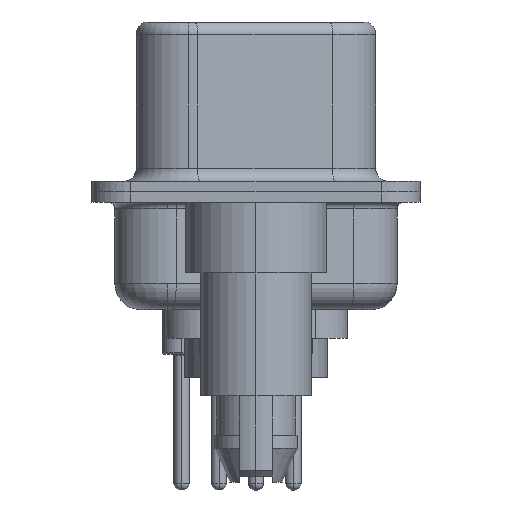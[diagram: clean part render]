
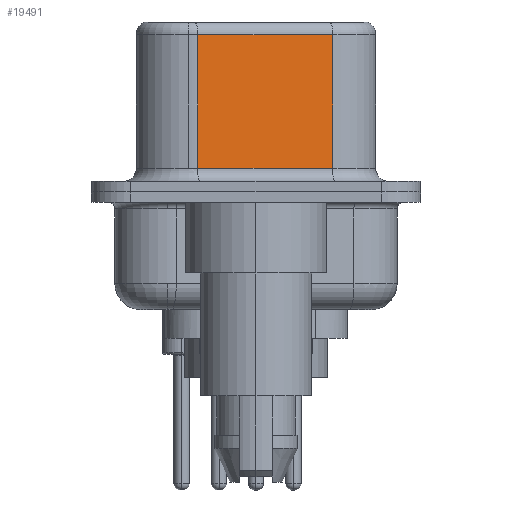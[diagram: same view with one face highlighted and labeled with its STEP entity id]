
A CAD part, left-side view. The second image highlights one B-rep face of the part: STEP entity #19491.
In plain terms, the highlighted planar face has unit normal (-0.985, -0.174, 0).
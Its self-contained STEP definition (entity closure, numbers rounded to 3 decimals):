
#1290 = VECTOR ( 'NONE', #22956, 1000. ) ;
#2112 = ORIENTED_EDGE ( 'NONE', *, *, #23496, .F. ) ;
#3891 = DIRECTION ( 'NONE',  ( 0., 0., -1. ) ) ;
#4011 = CARTESIAN_POINT ( 'NONE',  ( 4.585, -2.927, 6.02 ) ) ;
#4092 = VERTEX_POINT ( 'NONE', #12228 ) ;
#4845 = LINE ( 'NONE', #9576, #11020 ) ;
#5022 = EDGE_CURVE ( 'NONE', #10701, #4092, #4845, .T. ) ;
#5471 = LINE ( 'NONE', #13940, #19405 ) ;
#8380 = VERTEX_POINT ( 'NONE', #22483 ) ;
#9074 = CARTESIAN_POINT ( 'NONE',  ( 4.585, -2.927, 6.52 ) ) ;
#9576 = CARTESIAN_POINT ( 'NONE',  ( 4.585, -2.927, 6.02 ) ) ;
#10166 = EDGE_LOOP ( 'NONE', ( #2112, #16734, #15399, #18513 ) ) ;
#10701 = VERTEX_POINT ( 'NONE', #4011 ) ;
#11020 = VECTOR ( 'NONE', #21565, 1000. ) ;
#11113 = DIRECTION ( 'NONE',  ( 0.174, -0.985, 0. ) ) ;
#11999 = FACE_OUTER_BOUND ( 'NONE', #10166, .T. ) ;
#12228 = CARTESIAN_POINT ( 'NONE',  ( 3.675, 2.233, 6.02 ) ) ;
#13159 = EDGE_CURVE ( 'NONE', #4092, #19261, #5471, .T. ) ;
#13940 = CARTESIAN_POINT ( 'NONE',  ( 3.675, 2.233, 6.52 ) ) ;
#14363 = DIRECTION ( 'NONE',  ( -0.174, 0.985, 0. ) ) ;
#14646 = LINE ( 'NONE', #23168, #24270 ) ;
#14856 = AXIS2_PLACEMENT_3D ( 'NONE', #16352, #18273, #14363 ) ;
#15399 = ORIENTED_EDGE ( 'NONE', *, *, #13159, .T. ) ;
#16352 = CARTESIAN_POINT ( 'NONE',  ( 4.585, -2.927, 6.52 ) ) ;
#16734 = ORIENTED_EDGE ( 'NONE', *, *, #5022, .T. ) ;
#18273 = DIRECTION ( 'NONE',  ( 0.985, 0.174, 0. ) ) ;
#18513 = ORIENTED_EDGE ( 'NONE', *, *, #22863, .T. ) ;
#19261 = VERTEX_POINT ( 'NONE', #22584 ) ;
#19405 = VECTOR ( 'NONE', #3891, 1000. ) ;
#19491 = ADVANCED_FACE ( 'NONE', ( #11999 ), #19991, .F. ) ;
#19991 = PLANE ( 'NONE',  #14856 ) ;
#21565 = DIRECTION ( 'NONE',  ( -0.174, 0.985, 0. ) ) ;
#22483 = CARTESIAN_POINT ( 'NONE',  ( 4.585, -2.927, 0.9 ) ) ;
#22584 = CARTESIAN_POINT ( 'NONE',  ( 3.675, 2.233, 0.9 ) ) ;
#22863 = EDGE_CURVE ( 'NONE', #19261, #8380, #14646, .T. ) ;
#22956 = DIRECTION ( 'NONE',  ( 0., 0., -1. ) ) ;
#23168 = CARTESIAN_POINT ( 'NONE',  ( 4.585, -2.927, 0.9 ) ) ;
#23496 = EDGE_CURVE ( 'NONE', #10701, #8380, #24880, .T. ) ;
#24270 = VECTOR ( 'NONE', #11113, 1000. ) ;
#24880 = LINE ( 'NONE', #9074, #1290 ) ;
